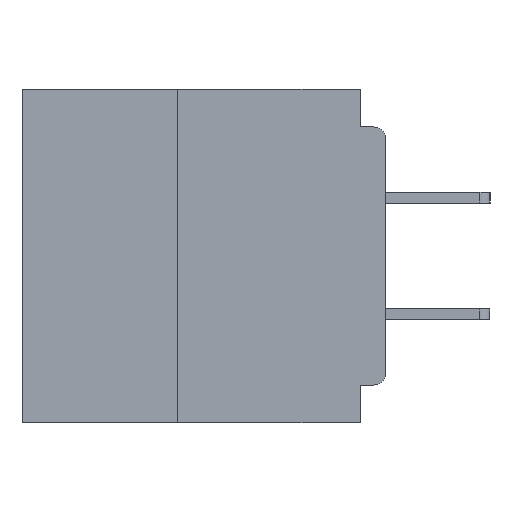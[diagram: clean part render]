
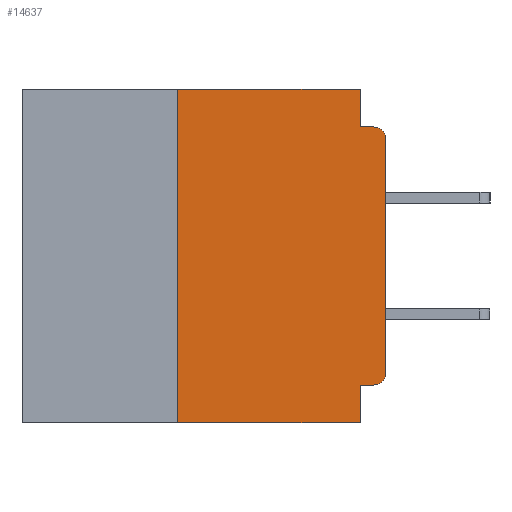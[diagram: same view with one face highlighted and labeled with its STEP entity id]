
A CAD part, left-side view. The second image highlights one B-rep face of the part: STEP entity #14637.
In plain terms, the highlighted planar face has unit normal (-1, 0, 0).
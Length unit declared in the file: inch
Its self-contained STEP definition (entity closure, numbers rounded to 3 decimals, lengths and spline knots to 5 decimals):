
#503 = EDGE_CURVE ( 'NONE', #15239, #19193, #37734, .T. ) ;
#770 = ORIENTED_EDGE ( 'NONE', *, *, #27428, .T. ) ;
#805 = ORIENTED_EDGE ( 'NONE', *, *, #503, .F. ) ;
#1737 = CARTESIAN_POINT ( 'NONE',  ( 0., 0.437, 0. ) ) ;
#2101 = ORIENTED_EDGE ( 'NONE', *, *, #21490, .F. ) ;
#3660 = DIRECTION ( 'NONE',  ( 0., -1., 0. ) ) ;
#5256 = CARTESIAN_POINT ( 'NONE',  ( 0., 0., 0. ) ) ;
#5343 = VERTEX_POINT ( 'NONE', #45729 ) ;
#5924 = EDGE_CURVE ( 'NONE', #6743, #9074, #43516, .T. ) ;
#6005 = VECTOR ( 'NONE', #24210, 39.37008 ) ;
#6743 = VERTEX_POINT ( 'NONE', #42335 ) ;
#8850 = CIRCLE ( 'NONE', #10321, 0.015 ) ;
#9074 = VERTEX_POINT ( 'NONE', #17091 ) ;
#9866 = DIRECTION ( 'NONE',  ( 0., 0., 1. ) ) ;
#10250 = CARTESIAN_POINT ( 'NONE',  ( 0., 0.25, -0.4 ) ) ;
#10321 = AXIS2_PLACEMENT_3D ( 'NONE', #54969, #27451, #59569 ) ;
#10961 = PLANE ( 'NONE',  #12073 ) ;
#11031 = CARTESIAN_POINT ( 'NONE',  ( 0., 0.031, -0.4 ) ) ;
#11088 = CARTESIAN_POINT ( 'NONE',  ( 0., 0.031, -0.4 ) ) ;
#11694 = VERTEX_POINT ( 'NONE', #11031 ) ;
#12015 = CARTESIAN_POINT ( 'NONE',  ( 0., 0., -0.34 ) ) ;
#12073 = AXIS2_PLACEMENT_3D ( 'NONE', #43374, #47996, #20319 ) ;
#12692 = CARTESIAN_POINT ( 'NONE',  ( 0., 0., -0.045 ) ) ;
#13785 = CARTESIAN_POINT ( 'NONE',  ( 0., 0.031, -0.355 ) ) ;
#14338 = VECTOR ( 'NONE', #52678, 39.37008 ) ;
#14637 = ADVANCED_FACE ( 'NONE', ( #32995 ), #10961, .F. ) ;
#14921 = VECTOR ( 'NONE', #49704, 39.37008 ) ;
#14947 = CARTESIAN_POINT ( 'NONE',  ( 0., 0.015, -0.355 ) ) ;
#15063 = EDGE_LOOP ( 'NONE', ( #770, #41577, #47808, #39688, #805, #50438, #19232, #28989, #2101, #28805 ) ) ;
#15239 = VERTEX_POINT ( 'NONE', #47531 ) ;
#17091 = CARTESIAN_POINT ( 'NONE',  ( 0., 0.015, -0.045 ) ) ;
#17574 = VERTEX_POINT ( 'NONE', #12015 ) ;
#19193 = VERTEX_POINT ( 'NONE', #27900 ) ;
#19232 = ORIENTED_EDGE ( 'NONE', *, *, #40839, .T. ) ;
#20319 = DIRECTION ( 'NONE',  ( 0., 0., -1. ) ) ;
#21490 = EDGE_CURVE ( 'NONE', #28943, #37692, #49618, .T. ) ;
#22417 = DIRECTION ( 'NONE',  ( -1., 0., 0. ) ) ;
#22501 = DIRECTION ( 'NONE',  ( 0., -1., 0. ) ) ;
#24210 = DIRECTION ( 'NONE',  ( 0., 0., -1. ) ) ;
#25090 = VECTOR ( 'NONE', #38455, 39.37008 ) ;
#26762 = LINE ( 'NONE', #11088, #14338 ) ;
#26935 = VECTOR ( 'NONE', #3660, 39.37008 ) ;
#27342 = LINE ( 'NONE', #12692, #14921 ) ;
#27428 = EDGE_CURVE ( 'NONE', #17574, #6743, #41261, .T. ) ;
#27451 = DIRECTION ( 'NONE',  ( -1., 0., 0. ) ) ;
#27900 = CARTESIAN_POINT ( 'NONE',  ( 0., 0.031, 0. ) ) ;
#28805 = ORIENTED_EDGE ( 'NONE', *, *, #53547, .T. ) ;
#28943 = VERTEX_POINT ( 'NONE', #14947 ) ;
#28989 = ORIENTED_EDGE ( 'NONE', *, *, #34627, .F. ) ;
#30630 = VECTOR ( 'NONE', #22501, 39.37008 ) ;
#32449 = CARTESIAN_POINT ( 'NONE',  ( 0., 0.25, -0.4 ) ) ;
#32995 = FACE_OUTER_BOUND ( 'NONE', #15063, .T. ) ;
#34627 = EDGE_CURVE ( 'NONE', #37692, #11694, #26762, .T. ) ;
#37530 = AXIS2_PLACEMENT_3D ( 'NONE', #50071, #22417, #54668 ) ;
#37692 = VERTEX_POINT ( 'NONE', #13785 ) ;
#37734 = LINE ( 'NONE', #1737, #26935 ) ;
#38455 = DIRECTION ( 'NONE',  ( 0., 1., 0. ) ) ;
#39688 = ORIENTED_EDGE ( 'NONE', *, *, #53102, .F. ) ;
#40839 = EDGE_CURVE ( 'NONE', #48609, #11694, #42862, .T. ) ;
#41261 = LINE ( 'NONE', #5256, #50576 ) ;
#41577 = ORIENTED_EDGE ( 'NONE', *, *, #5924, .T. ) ;
#41908 = VECTOR ( 'NONE', #42679, 39.37008 ) ;
#42335 = CARTESIAN_POINT ( 'NONE',  ( 0., 0., -0.06 ) ) ;
#42679 = DIRECTION ( 'NONE',  ( 0., 0., 1. ) ) ;
#42862 = LINE ( 'NONE', #54541, #30630 ) ;
#42959 = LINE ( 'NONE', #56429, #6005 ) ;
#43374 = CARTESIAN_POINT ( 'NONE',  ( 0., 0.437, 0. ) ) ;
#43516 = CIRCLE ( 'NONE', #37530, 0.015 ) ;
#45729 = CARTESIAN_POINT ( 'NONE',  ( 0., 0.031, -0.045 ) ) ;
#46962 = EDGE_CURVE ( 'NONE', #48609, #15239, #51215, .T. ) ;
#47531 = CARTESIAN_POINT ( 'NONE',  ( 0., 0.25, 0. ) ) ;
#47808 = ORIENTED_EDGE ( 'NONE', *, *, #59350, .F. ) ;
#47903 = CARTESIAN_POINT ( 'NONE',  ( 0., 0., -0.355 ) ) ;
#47996 = DIRECTION ( 'NONE',  ( 1., 0., 0. ) ) ;
#48609 = VERTEX_POINT ( 'NONE', #32449 ) ;
#49618 = LINE ( 'NONE', #47903, #25090 ) ;
#49704 = DIRECTION ( 'NONE',  ( 0., -1., 0. ) ) ;
#50071 = CARTESIAN_POINT ( 'NONE',  ( 0., 0.015, -0.06 ) ) ;
#50438 = ORIENTED_EDGE ( 'NONE', *, *, #46962, .F. ) ;
#50576 = VECTOR ( 'NONE', #9866, 39.37008 ) ;
#51215 = LINE ( 'NONE', #10250, #41908 ) ;
#52678 = DIRECTION ( 'NONE',  ( 0., 0., -1. ) ) ;
#53102 = EDGE_CURVE ( 'NONE', #19193, #5343, #42959, .T. ) ;
#53547 = EDGE_CURVE ( 'NONE', #28943, #17574, #8850, .T. ) ;
#54541 = CARTESIAN_POINT ( 'NONE',  ( 0., 0.437, -0.4 ) ) ;
#54668 = DIRECTION ( 'NONE',  ( 0., 0., -1. ) ) ;
#54969 = CARTESIAN_POINT ( 'NONE',  ( 0., 0.015, -0.34 ) ) ;
#56429 = CARTESIAN_POINT ( 'NONE',  ( 0., 0.031, 0. ) ) ;
#59350 = EDGE_CURVE ( 'NONE', #5343, #9074, #27342, .T. ) ;
#59569 = DIRECTION ( 'NONE',  ( 0., 0., -1. ) ) ;
